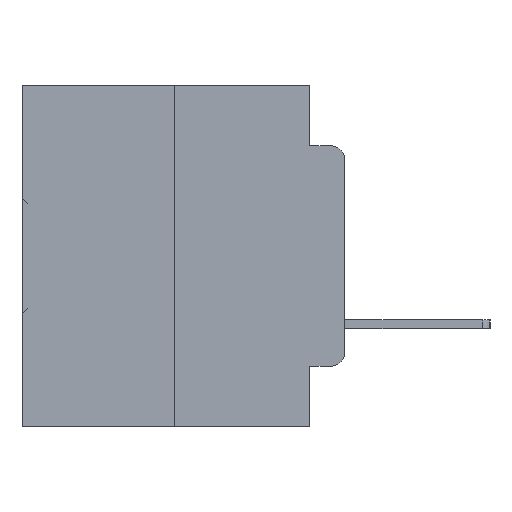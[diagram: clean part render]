
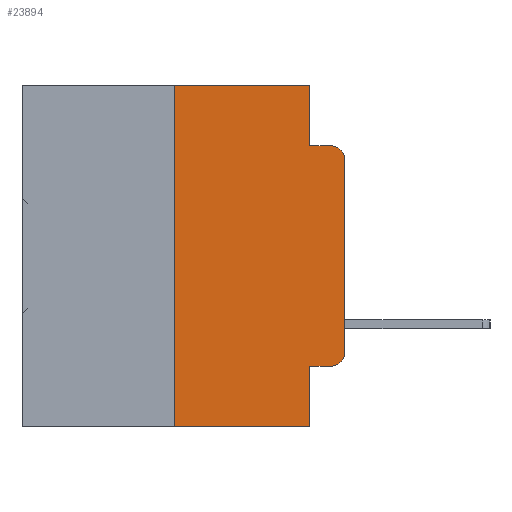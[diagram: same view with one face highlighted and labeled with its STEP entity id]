
A CAD part, left-side view. The second image highlights one B-rep face of the part: STEP entity #23894.
In plain terms, the highlighted planar face has unit normal (-1, 0, 0).
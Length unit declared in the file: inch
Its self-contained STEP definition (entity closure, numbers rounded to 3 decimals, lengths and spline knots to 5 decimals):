
#184 = DIRECTION ( 'NONE',  ( 0., 0., -1. ) ) ;
#300 = CARTESIAN_POINT ( 'NONE',  ( 0., 0.051, 0. ) ) ;
#447 = CARTESIAN_POINT ( 'NONE',  ( 0., 0.25, 0. ) ) ;
#814 = DIRECTION ( 'NONE',  ( 0., -1., 0. ) ) ;
#877 = AXIS2_PLACEMENT_3D ( 'NONE', #1146, #28543, #12190 ) ;
#1146 = CARTESIAN_POINT ( 'NONE',  ( 0., 0.473, 0. ) ) ;
#1170 = CARTESIAN_POINT ( 'NONE',  ( 0., 0.051, -0.0885 ) ) ;
#1279 = CARTESIAN_POINT ( 'NONE',  ( 0., 0.02, -0.4115 ) ) ;
#1402 = CARTESIAN_POINT ( 'NONE',  ( 0., 0.051, -0.5 ) ) ;
#1816 = EDGE_CURVE ( 'NONE', #32137, #16525, #21155, .T. ) ;
#3636 = EDGE_CURVE ( 'NONE', #14765, #32137, #31299, .T. ) ;
#4064 = VECTOR ( 'NONE', #28849, 39.37008 ) ;
#4182 = CARTESIAN_POINT ( 'NONE',  ( 0., 0.473, -0.5 ) ) ;
#5015 = CARTESIAN_POINT ( 'NONE',  ( 0., 0.051, -0.4115 ) ) ;
#5236 = CARTESIAN_POINT ( 'NONE',  ( 0., 0.051, 0. ) ) ;
#5837 = CARTESIAN_POINT ( 'NONE',  ( 0., 0.02, -0.3915 ) ) ;
#7841 = VERTEX_POINT ( 'NONE', #1170 ) ;
#8625 = DIRECTION ( 'NONE',  ( 0., 0., -1. ) ) ;
#8877 = DIRECTION ( 'NONE',  ( 0., -1., 0. ) ) ;
#9193 = EDGE_CURVE ( 'NONE', #14765, #32154, #34253, .T. ) ;
#9256 = CARTESIAN_POINT ( 'NONE',  ( 0., 0., -0.3915 ) ) ;
#10102 = ORIENTED_EDGE ( 'NONE', *, *, #22460, .T. ) ;
#10341 = VECTOR ( 'NONE', #8877, 39.37008 ) ;
#10734 = DIRECTION ( 'NONE',  ( 0., 0., 1. ) ) ;
#10989 = LINE ( 'NONE', #33602, #31941 ) ;
#11031 = EDGE_CURVE ( 'NONE', #11186, #17643, #29279, .T. ) ;
#11056 = CARTESIAN_POINT ( 'NONE',  ( 0., 0., -0.1085 ) ) ;
#11186 = VERTEX_POINT ( 'NONE', #30579 ) ;
#11607 = VECTOR ( 'NONE', #26007, 39.37008 ) ;
#11837 = CARTESIAN_POINT ( 'NONE',  ( 0., 0., 0. ) ) ;
#12190 = DIRECTION ( 'NONE',  ( 0., 0., -1. ) ) ;
#12869 = EDGE_CURVE ( 'NONE', #16888, #7841, #28276, .T. ) ;
#13203 = EDGE_LOOP ( 'NONE', ( #26315, #15168, #22418, #23738, #17314, #16051, #10102, #35311, #22485, #23337 ) ) ;
#14711 = VECTOR ( 'NONE', #19756, 39.37008 ) ;
#14765 = VERTEX_POINT ( 'NONE', #5015 ) ;
#15168 = ORIENTED_EDGE ( 'NONE', *, *, #21981, .T. ) ;
#15978 = DIRECTION ( 'NONE',  ( -1., 0., 0. ) ) ;
#16051 = ORIENTED_EDGE ( 'NONE', *, *, #11031, .F. ) ;
#16525 = VERTEX_POINT ( 'NONE', #9256 ) ;
#16641 = AXIS2_PLACEMENT_3D ( 'NONE', #32356, #15978, #35094 ) ;
#16888 = VERTEX_POINT ( 'NONE', #5236 ) ;
#17020 = CARTESIAN_POINT ( 'NONE',  ( 0., 0.473, 0. ) ) ;
#17202 = VERTEX_POINT ( 'NONE', #17545 ) ;
#17314 = ORIENTED_EDGE ( 'NONE', *, *, #22235, .F. ) ;
#17545 = CARTESIAN_POINT ( 'NONE',  ( 0., 0.02, -0.0885 ) ) ;
#17643 = VERTEX_POINT ( 'NONE', #447 ) ;
#17708 = CARTESIAN_POINT ( 'NONE',  ( 0., 0.051, 0. ) ) ;
#19756 = DIRECTION ( 'NONE',  ( 0., -1., 0. ) ) ;
#20142 = EDGE_CURVE ( 'NONE', #7841, #17202, #10989, .T. ) ;
#21155 = CIRCLE ( 'NONE', #29005, 0.02 ) ;
#21967 = VECTOR ( 'NONE', #10734, 39.37008 ) ;
#21981 = EDGE_CURVE ( 'NONE', #29496, #17202, #30587, .T. ) ;
#22235 = EDGE_CURVE ( 'NONE', #17643, #16888, #24553, .T. ) ;
#22382 = LINE ( 'NONE', #4182, #4064 ) ;
#22418 = ORIENTED_EDGE ( 'NONE', *, *, #20142, .F. ) ;
#22460 = EDGE_CURVE ( 'NONE', #11186, #32154, #22382, .T. ) ;
#22464 = CARTESIAN_POINT ( 'NONE',  ( 0., 0.051, -0.4115 ) ) ;
#22485 = ORIENTED_EDGE ( 'NONE', *, *, #3636, .T. ) ;
#23337 = ORIENTED_EDGE ( 'NONE', *, *, #1816, .T. ) ;
#23738 = ORIENTED_EDGE ( 'NONE', *, *, #12869, .F. ) ;
#23834 = EDGE_CURVE ( 'NONE', #16525, #29496, #25703, .T. ) ;
#23894 = ADVANCED_FACE ( 'NONE', ( #30404 ), #28426, .F. ) ;
#24231 = CARTESIAN_POINT ( 'NONE',  ( 0., 0.25, 0. ) ) ;
#24553 = LINE ( 'NONE', #17020, #14711 ) ;
#24998 = DIRECTION ( 'NONE',  ( -1., 0., 0. ) ) ;
#25703 = LINE ( 'NONE', #11837, #32103 ) ;
#26007 = DIRECTION ( 'NONE',  ( 0., 0., -1. ) ) ;
#26315 = ORIENTED_EDGE ( 'NONE', *, *, #23834, .T. ) ;
#28276 = LINE ( 'NONE', #300, #29136 ) ;
#28426 = PLANE ( 'NONE',  #877 ) ;
#28543 = DIRECTION ( 'NONE',  ( 1., 0., 0. ) ) ;
#28849 = DIRECTION ( 'NONE',  ( 0., -1., 0. ) ) ;
#29005 = AXIS2_PLACEMENT_3D ( 'NONE', #5837, #24998, #8625 ) ;
#29136 = VECTOR ( 'NONE', #184, 39.37008 ) ;
#29279 = LINE ( 'NONE', #24231, #21967 ) ;
#29496 = VERTEX_POINT ( 'NONE', #11056 ) ;
#30404 = FACE_OUTER_BOUND ( 'NONE', #13203, .T. ) ;
#30579 = CARTESIAN_POINT ( 'NONE',  ( 0., 0.25, -0.5 ) ) ;
#30587 = CIRCLE ( 'NONE', #16641, 0.02 ) ;
#31299 = LINE ( 'NONE', #22464, #10341 ) ;
#31941 = VECTOR ( 'NONE', #814, 39.37008 ) ;
#32103 = VECTOR ( 'NONE', #33694, 39.37008 ) ;
#32137 = VERTEX_POINT ( 'NONE', #1279 ) ;
#32154 = VERTEX_POINT ( 'NONE', #1402 ) ;
#32356 = CARTESIAN_POINT ( 'NONE',  ( 0., 0.02, -0.1085 ) ) ;
#33602 = CARTESIAN_POINT ( 'NONE',  ( 0., 0.051, -0.0885 ) ) ;
#33694 = DIRECTION ( 'NONE',  ( 0., 0., 1. ) ) ;
#34253 = LINE ( 'NONE', #17708, #11607 ) ;
#35094 = DIRECTION ( 'NONE',  ( 0., 0., -1. ) ) ;
#35311 = ORIENTED_EDGE ( 'NONE', *, *, #9193, .F. ) ;
